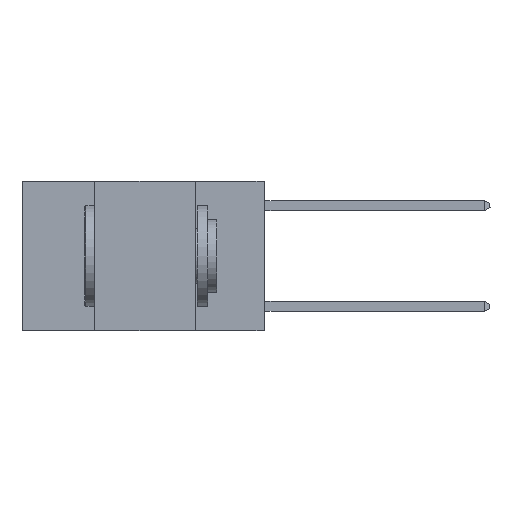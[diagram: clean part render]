
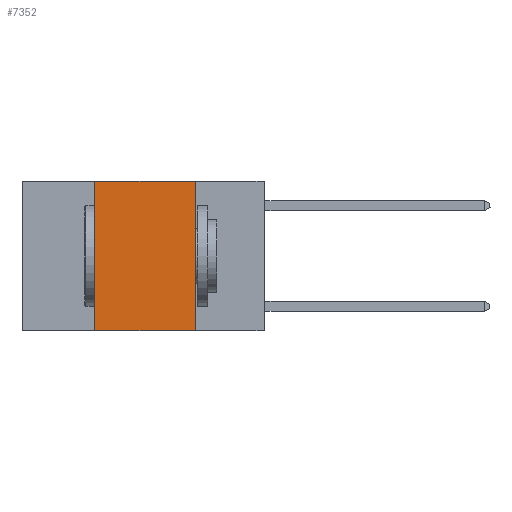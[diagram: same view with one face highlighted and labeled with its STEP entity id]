
A CAD part, left-side view. The second image highlights one B-rep face of the part: STEP entity #7352.
In plain terms, the highlighted planar face has unit normal (-1, 0, 0).
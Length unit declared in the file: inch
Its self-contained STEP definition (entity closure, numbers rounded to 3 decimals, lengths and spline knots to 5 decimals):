
#183 = ORIENTED_EDGE ( 'NONE', *, *, #15816, .F. ) ;
#1618 = FACE_OUTER_BOUND ( 'NONE', #8765, .T. ) ;
#1714 = VERTEX_POINT ( 'NONE', #7244 ) ;
#2129 = DIRECTION ( 'NONE',  ( 0., -1., 0. ) ) ;
#2252 = VERTEX_POINT ( 'NONE', #19736 ) ;
#3045 = LINE ( 'NONE', #9785, #6678 ) ;
#3273 = LINE ( 'NONE', #11495, #15090 ) ;
#3317 = ORIENTED_EDGE ( 'NONE', *, *, #13736, .F. ) ;
#3884 = VERTEX_POINT ( 'NONE', #4892 ) ;
#4280 = ORIENTED_EDGE ( 'NONE', *, *, #17874, .T. ) ;
#4293 = EDGE_CURVE ( 'NONE', #1714, #3884, #12986, .T. ) ;
#4892 = CARTESIAN_POINT ( 'NONE',  ( 0., 0.17, 0. ) ) ;
#5300 = AXIS2_PLACEMENT_3D ( 'NONE', #17661, #8398, #19201 ) ;
#5322 = PLANE ( 'NONE',  #5300 ) ;
#5449 = DIRECTION ( 'NONE',  ( 0., 0., -1. ) ) ;
#6417 = CARTESIAN_POINT ( 'NONE',  ( 0., 0.42, 0. ) ) ;
#6678 = VECTOR ( 'NONE', #2129, 39.37008 ) ;
#7244 = CARTESIAN_POINT ( 'NONE',  ( 0., 0.42, 0. ) ) ;
#7352 = ADVANCED_FACE ( 'NONE', ( #1618 ), #5322, .F. ) ;
#8398 = DIRECTION ( 'NONE',  ( 1., 0., 0. ) ) ;
#8765 = EDGE_LOOP ( 'NONE', ( #3317, #16115, #183, #4280 ) ) ;
#8851 = VECTOR ( 'NONE', #10729, 39.37008 ) ;
#9148 = VERTEX_POINT ( 'NONE', #19170 ) ;
#9785 = CARTESIAN_POINT ( 'NONE',  ( 0., 0.6, -0.37 ) ) ;
#10655 = LINE ( 'NONE', #6417, #14256 ) ;
#10729 = DIRECTION ( 'NONE',  ( 0., -1., 0. ) ) ;
#11495 = CARTESIAN_POINT ( 'NONE',  ( 0., 0.17, 0. ) ) ;
#12986 = LINE ( 'NONE', #13755, #8851 ) ;
#13736 = EDGE_CURVE ( 'NONE', #3884, #2252, #3273, .T. ) ;
#13755 = CARTESIAN_POINT ( 'NONE',  ( 0., 0.6, 0. ) ) ;
#14256 = VECTOR ( 'NONE', #18725, 39.37008 ) ;
#15090 = VECTOR ( 'NONE', #5449, 39.37008 ) ;
#15816 = EDGE_CURVE ( 'NONE', #9148, #1714, #10655, .T. ) ;
#16115 = ORIENTED_EDGE ( 'NONE', *, *, #4293, .F. ) ;
#17661 = CARTESIAN_POINT ( 'NONE',  ( 0., 0.6, 0. ) ) ;
#17874 = EDGE_CURVE ( 'NONE', #9148, #2252, #3045, .T. ) ;
#18725 = DIRECTION ( 'NONE',  ( 0., 0., 1. ) ) ;
#19170 = CARTESIAN_POINT ( 'NONE',  ( 0., 0.42, -0.37 ) ) ;
#19201 = DIRECTION ( 'NONE',  ( 0., 0., -1. ) ) ;
#19736 = CARTESIAN_POINT ( 'NONE',  ( 0., 0.17, -0.37 ) ) ;
